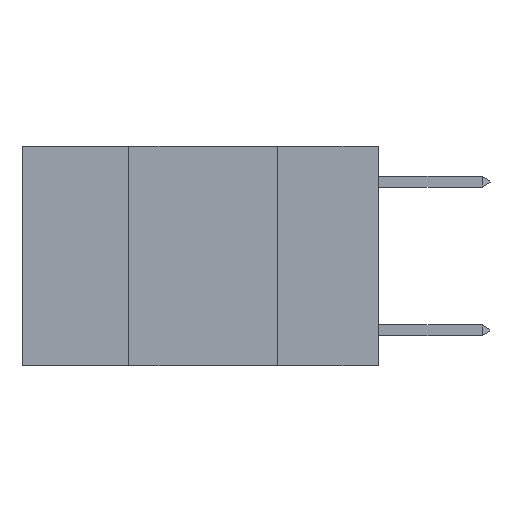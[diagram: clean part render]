
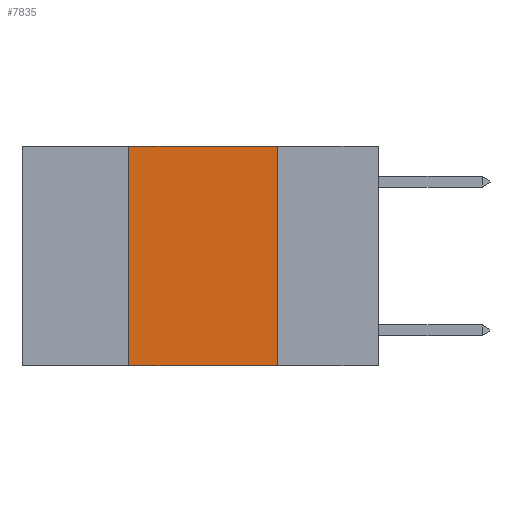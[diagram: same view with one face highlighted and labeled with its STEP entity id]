
A CAD part, left-side view. The second image highlights one B-rep face of the part: STEP entity #7835.
In plain terms, the highlighted planar face has unit normal (-1, 0, 0).
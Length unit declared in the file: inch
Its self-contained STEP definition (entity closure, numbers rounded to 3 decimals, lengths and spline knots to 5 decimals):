
#708 = CARTESIAN_POINT ( 'NONE',  ( 0., 0.42, 0. ) ) ;
#763 = DIRECTION ( 'NONE',  ( 0., -1., 0. ) ) ;
#808 = VECTOR ( 'NONE', #8531, 39.37008 ) ;
#1067 = VECTOR ( 'NONE', #6747, 39.37008 ) ;
#1308 = ORIENTED_EDGE ( 'NONE', *, *, #3928, .F. ) ;
#1372 = EDGE_CURVE ( 'NONE', #7016, #3882, #4516, .T. ) ;
#2181 = CARTESIAN_POINT ( 'NONE',  ( 0., 0.6, 0. ) ) ;
#2295 = EDGE_LOOP ( 'NONE', ( #4584, #1308, #4298, #5965 ) ) ;
#2458 = CARTESIAN_POINT ( 'NONE',  ( 0., 0.42, 0. ) ) ;
#3251 = CARTESIAN_POINT ( 'NONE',  ( 0., 0.6, 0. ) ) ;
#3407 = DIRECTION ( 'NONE',  ( 0., 0., 1. ) ) ;
#3622 = LINE ( 'NONE', #6006, #1067 ) ;
#3782 = EDGE_CURVE ( 'NONE', #7016, #6831, #9951, .T. ) ;
#3878 = VECTOR ( 'NONE', #763, 39.37008 ) ;
#3882 = VERTEX_POINT ( 'NONE', #2458 ) ;
#3928 = EDGE_CURVE ( 'NONE', #3882, #8399, #6919, .T. ) ;
#4298 = ORIENTED_EDGE ( 'NONE', *, *, #1372, .F. ) ;
#4506 = DIRECTION ( 'NONE',  ( 0., 0., -1. ) ) ;
#4516 = LINE ( 'NONE', #708, #6494 ) ;
#4584 = ORIENTED_EDGE ( 'NONE', *, *, #9746, .F. ) ;
#5131 = CARTESIAN_POINT ( 'NONE',  ( 0., 0.17, 0. ) ) ;
#5393 = CARTESIAN_POINT ( 'NONE',  ( 0., 0.6, -0.37 ) ) ;
#5965 = ORIENTED_EDGE ( 'NONE', *, *, #3782, .T. ) ;
#6006 = CARTESIAN_POINT ( 'NONE',  ( 0., 0.17, 0. ) ) ;
#6494 = VECTOR ( 'NONE', #3407, 39.37008 ) ;
#6690 = CARTESIAN_POINT ( 'NONE',  ( 0., 0.17, -0.37 ) ) ;
#6747 = DIRECTION ( 'NONE',  ( 0., 0., -1. ) ) ;
#6831 = VERTEX_POINT ( 'NONE', #6690 ) ;
#6919 = LINE ( 'NONE', #3251, #808 ) ;
#7016 = VERTEX_POINT ( 'NONE', #8353 ) ;
#7628 = FACE_OUTER_BOUND ( 'NONE', #2295, .T. ) ;
#7835 = ADVANCED_FACE ( 'NONE', ( #7628 ), #8255, .F. ) ;
#8255 = PLANE ( 'NONE',  #9961 ) ;
#8353 = CARTESIAN_POINT ( 'NONE',  ( 0., 0.42, -0.37 ) ) ;
#8399 = VERTEX_POINT ( 'NONE', #5131 ) ;
#8531 = DIRECTION ( 'NONE',  ( 0., -1., 0. ) ) ;
#9044 = DIRECTION ( 'NONE',  ( 1., 0., 0. ) ) ;
#9746 = EDGE_CURVE ( 'NONE', #8399, #6831, #3622, .T. ) ;
#9951 = LINE ( 'NONE', #5393, #3878 ) ;
#9961 = AXIS2_PLACEMENT_3D ( 'NONE', #2181, #9044, #4506 ) ;
